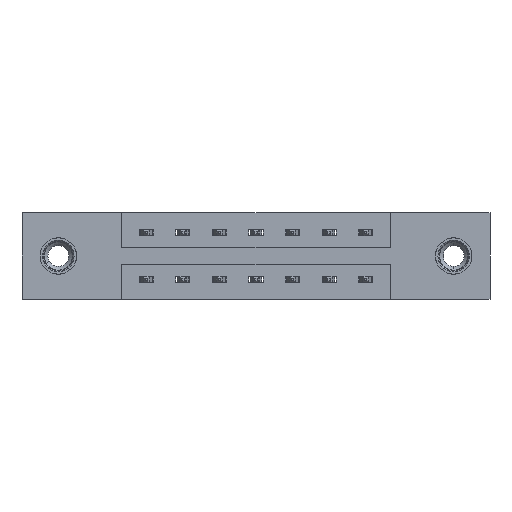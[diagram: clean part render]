
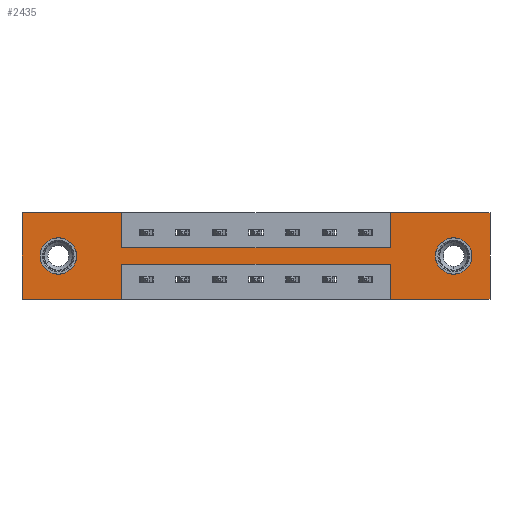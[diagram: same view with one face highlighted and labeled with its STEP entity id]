
A CAD part, front view. The second image highlights one B-rep face of the part: STEP entity #2435.
In plain terms, the highlighted planar face has unit normal (0, -1, 0).
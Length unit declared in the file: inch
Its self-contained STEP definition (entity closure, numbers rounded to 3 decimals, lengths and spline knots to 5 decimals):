
#103 = PLANE ( 'NONE',  #8969 ) ;
#234 = DIRECTION ( 'NONE',  ( 0., 0., 1. ) ) ;
#353 = DIRECTION ( 'NONE',  ( -1., 0., 0. ) ) ;
#356 = CIRCLE ( 'NONE', #10719, 0.078 ) ;
#375 = EDGE_CURVE ( 'NONE', #5994, #7460, #5939, .T. ) ;
#381 = CARTESIAN_POINT ( 'NONE',  ( 0.425, 0., -0.22 ) ) ;
#411 = CARTESIAN_POINT ( 'NONE',  ( 1.843, 0., -0.185 ) ) ;
#418 = EDGE_CURVE ( 'NONE', #3262, #6279, #932, .T. ) ;
#466 = LINE ( 'NONE', #6577, #4883 ) ;
#505 = EDGE_CURVE ( 'NONE', #6763, #5525, #2140, .T. ) ;
#507 = DIRECTION ( 'NONE',  ( 0., -1., 0. ) ) ;
#521 = CARTESIAN_POINT ( 'NONE',  ( 0., 0., -0.37 ) ) ;
#534 = EDGE_CURVE ( 'NONE', #8706, #6865, #11055, .T. ) ;
#595 = AXIS2_PLACEMENT_3D ( 'NONE', #2732, #8881, #3634 ) ;
#843 = EDGE_CURVE ( 'NONE', #5814, #2511, #7992, .T. ) ;
#901 = DIRECTION ( 'NONE',  ( -1., 0., 0. ) ) ;
#932 = LINE ( 'NONE', #4922, #3001 ) ;
#967 = DIRECTION ( 'NONE',  ( 0., 0., -1. ) ) ;
#1188 = VECTOR ( 'NONE', #1465, 39.37008 ) ;
#1202 = CARTESIAN_POINT ( 'NONE',  ( 0.425, 0., -0.15 ) ) ;
#1412 = LINE ( 'NONE', #10168, #8451 ) ;
#1465 = DIRECTION ( 'NONE',  ( -1., 0., 0. ) ) ;
#1551 = CARTESIAN_POINT ( 'NONE',  ( 0., 0., -0.37 ) ) ;
#1708 = ORIENTED_EDGE ( 'NONE', *, *, #534, .F. ) ;
#2140 = CIRCLE ( 'NONE', #7482, 0.078 ) ;
#2142 = CARTESIAN_POINT ( 'NONE',  ( 0., 0., 0. ) ) ;
#2435 = ADVANCED_FACE ( 'NONE', ( #4099, #6209, #8510 ), #103, .T. ) ;
#2511 = VERTEX_POINT ( 'NONE', #2798 ) ;
#2574 = CARTESIAN_POINT ( 'NONE',  ( 1.573, 0., -0.37 ) ) ;
#2670 = LINE ( 'NONE', #7163, #5349 ) ;
#2690 = CARTESIAN_POINT ( 'NONE',  ( 0.155, 0., -0.107 ) ) ;
#2714 = DIRECTION ( 'NONE',  ( 1., 0., 0. ) ) ;
#2716 = EDGE_LOOP ( 'NONE', ( #4762, #5065, #7401, #9607, #5332, #8219, #10369, #10618, #1708, #4637, #6989, #7256 ) ) ;
#2732 = CARTESIAN_POINT ( 'NONE',  ( 0.155, 0., -0.185 ) ) ;
#2735 = VERTEX_POINT ( 'NONE', #2142 ) ;
#2763 = CARTESIAN_POINT ( 'NONE',  ( 0.155, 0., -0.185 ) ) ;
#2777 = DIRECTION ( 'NONE',  ( 0., 0., -1. ) ) ;
#2798 = CARTESIAN_POINT ( 'NONE',  ( 0., 0., -0.37 ) ) ;
#2953 = VERTEX_POINT ( 'NONE', #2690 ) ;
#3001 = VECTOR ( 'NONE', #5689, 39.37008 ) ;
#3045 = VECTOR ( 'NONE', #234, 39.37008 ) ;
#3068 = VERTEX_POINT ( 'NONE', #2574 ) ;
#3210 = CARTESIAN_POINT ( 'NONE',  ( 1.573, 0., -0.15 ) ) ;
#3262 = VERTEX_POINT ( 'NONE', #8260 ) ;
#3384 = DIRECTION ( 'NONE',  ( 0., 0., -1. ) ) ;
#3387 = EDGE_CURVE ( 'NONE', #2735, #8706, #2670, .T. ) ;
#3389 = DIRECTION ( 'NONE',  ( 0., 0., -1. ) ) ;
#3492 = CARTESIAN_POINT ( 'NONE',  ( 0., 0., 0. ) ) ;
#3539 = EDGE_CURVE ( 'NONE', #6865, #8685, #6042, .T. ) ;
#3597 = CIRCLE ( 'NONE', #10507, 0.078 ) ;
#3634 = DIRECTION ( 'NONE',  ( 0., 0., 1. ) ) ;
#3670 = DIRECTION ( 'NONE',  ( 0., 0., 1. ) ) ;
#3967 = EDGE_CURVE ( 'NONE', #7460, #5814, #10506, .T. ) ;
#4099 = FACE_BOUND ( 'NONE', #5236, .T. ) ;
#4181 = CARTESIAN_POINT ( 'NONE',  ( 1.843, 0., -0.185 ) ) ;
#4633 = LINE ( 'NONE', #7412, #11146 ) ;
#4637 = ORIENTED_EDGE ( 'NONE', *, *, #3387, .F. ) ;
#4762 = ORIENTED_EDGE ( 'NONE', *, *, #3967, .F. ) ;
#4883 = VECTOR ( 'NONE', #10585, 39.37008 ) ;
#4922 = CARTESIAN_POINT ( 'NONE',  ( 1.998, 0., 0. ) ) ;
#5016 = CARTESIAN_POINT ( 'NONE',  ( 0.425, 0., -0.15 ) ) ;
#5065 = ORIENTED_EDGE ( 'NONE', *, *, #375, .F. ) ;
#5093 = DIRECTION ( 'NONE',  ( 0., 0., -1. ) ) ;
#5137 = VERTEX_POINT ( 'NONE', #10341 ) ;
#5236 = EDGE_LOOP ( 'NONE', ( #10238, #8347 ) ) ;
#5293 = DIRECTION ( 'NONE',  ( 1., 0., 0. ) ) ;
#5332 = ORIENTED_EDGE ( 'NONE', *, *, #418, .F. ) ;
#5349 = VECTOR ( 'NONE', #2714, 39.37008 ) ;
#5423 = LINE ( 'NONE', #7278, #3045 ) ;
#5525 = VERTEX_POINT ( 'NONE', #6685 ) ;
#5689 = DIRECTION ( 'NONE',  ( 0., 0., -1. ) ) ;
#5747 = EDGE_CURVE ( 'NONE', #2511, #2735, #466, .T. ) ;
#5814 = VERTEX_POINT ( 'NONE', #8512 ) ;
#5864 = EDGE_CURVE ( 'NONE', #3068, #5994, #1412, .T. ) ;
#5939 = LINE ( 'NONE', #381, #10160 ) ;
#5994 = VERTEX_POINT ( 'NONE', #10668 ) ;
#6042 = LINE ( 'NONE', #1202, #10256 ) ;
#6209 = FACE_BOUND ( 'NONE', #8548, .T. ) ;
#6279 = VERTEX_POINT ( 'NONE', #7762 ) ;
#6298 = ORIENTED_EDGE ( 'NONE', *, *, #9656, .T. ) ;
#6348 = VECTOR ( 'NONE', #3389, 39.37008 ) ;
#6543 = CIRCLE ( 'NONE', #595, 0.078 ) ;
#6549 = EDGE_CURVE ( 'NONE', #7294, #2953, #3597, .T. ) ;
#6577 = CARTESIAN_POINT ( 'NONE',  ( 0., 0., 0. ) ) ;
#6606 = EDGE_CURVE ( 'NONE', #8685, #5137, #5423, .T. ) ;
#6631 = CARTESIAN_POINT ( 'NONE',  ( 0.425, 0., -0.22 ) ) ;
#6685 = CARTESIAN_POINT ( 'NONE',  ( 1.843, 0., -0.107 ) ) ;
#6763 = VERTEX_POINT ( 'NONE', #9163 ) ;
#6865 = VERTEX_POINT ( 'NONE', #5016 ) ;
#6989 = ORIENTED_EDGE ( 'NONE', *, *, #5747, .F. ) ;
#7091 = VECTOR ( 'NONE', #5293, 39.37008 ) ;
#7163 = CARTESIAN_POINT ( 'NONE',  ( 0., 0., 0. ) ) ;
#7256 = ORIENTED_EDGE ( 'NONE', *, *, #843, .F. ) ;
#7278 = CARTESIAN_POINT ( 'NONE',  ( 1.573, 0., 0. ) ) ;
#7294 = VERTEX_POINT ( 'NONE', #7301 ) ;
#7301 = CARTESIAN_POINT ( 'NONE',  ( 0.155, 0., -0.263 ) ) ;
#7401 = ORIENTED_EDGE ( 'NONE', *, *, #5864, .F. ) ;
#7412 = CARTESIAN_POINT ( 'NONE',  ( 0., 0., -0.37 ) ) ;
#7416 = DIRECTION ( 'NONE',  ( 0., 1., 0. ) ) ;
#7460 = VERTEX_POINT ( 'NONE', #6631 ) ;
#7482 = AXIS2_PLACEMENT_3D ( 'NONE', #411, #7416, #3384 ) ;
#7762 = CARTESIAN_POINT ( 'NONE',  ( 1.998, 0., -0.37 ) ) ;
#7925 = DIRECTION ( 'NONE',  ( 1., 0., 0. ) ) ;
#7992 = LINE ( 'NONE', #1551, #1188 ) ;
#8062 = CARTESIAN_POINT ( 'NONE',  ( 0.425, 0., -0.37 ) ) ;
#8219 = ORIENTED_EDGE ( 'NONE', *, *, #9571, .F. ) ;
#8260 = CARTESIAN_POINT ( 'NONE',  ( 1.998, 0., 0. ) ) ;
#8347 = ORIENTED_EDGE ( 'NONE', *, *, #505, .T. ) ;
#8451 = VECTOR ( 'NONE', #11130, 39.37008 ) ;
#8493 = CARTESIAN_POINT ( 'NONE',  ( 0.425, 0., 0. ) ) ;
#8510 = FACE_OUTER_BOUND ( 'NONE', #2716, .T. ) ;
#8512 = CARTESIAN_POINT ( 'NONE',  ( 0.425, 0., -0.37 ) ) ;
#8542 = EDGE_CURVE ( 'NONE', #6279, #3068, #4633, .T. ) ;
#8548 = EDGE_LOOP ( 'NONE', ( #6298, #10744 ) ) ;
#8685 = VERTEX_POINT ( 'NONE', #3210 ) ;
#8706 = VERTEX_POINT ( 'NONE', #8493 ) ;
#8735 = EDGE_CURVE ( 'NONE', #5525, #6763, #356, .T. ) ;
#8881 = DIRECTION ( 'NONE',  ( 0., 1., 0. ) ) ;
#8901 = DIRECTION ( 'NONE',  ( 0., 1., 0. ) ) ;
#8969 = AXIS2_PLACEMENT_3D ( 'NONE', #521, #507, #2777 ) ;
#9163 = CARTESIAN_POINT ( 'NONE',  ( 1.843, 0., -0.263 ) ) ;
#9332 = LINE ( 'NONE', #3492, #7091 ) ;
#9571 = EDGE_CURVE ( 'NONE', #5137, #3262, #9332, .T. ) ;
#9607 = ORIENTED_EDGE ( 'NONE', *, *, #8542, .F. ) ;
#9656 = EDGE_CURVE ( 'NONE', #2953, #7294, #6543, .T. ) ;
#10160 = VECTOR ( 'NONE', #901, 39.37008 ) ;
#10168 = CARTESIAN_POINT ( 'NONE',  ( 1.573, 0., -0.37 ) ) ;
#10182 = DIRECTION ( 'NONE',  ( 0., 1., 0. ) ) ;
#10238 = ORIENTED_EDGE ( 'NONE', *, *, #8735, .T. ) ;
#10246 = VECTOR ( 'NONE', #967, 39.37008 ) ;
#10256 = VECTOR ( 'NONE', #7925, 39.37008 ) ;
#10341 = CARTESIAN_POINT ( 'NONE',  ( 1.573, 0., 0. ) ) ;
#10369 = ORIENTED_EDGE ( 'NONE', *, *, #6606, .F. ) ;
#10506 = LINE ( 'NONE', #8062, #10246 ) ;
#10507 = AXIS2_PLACEMENT_3D ( 'NONE', #2763, #8901, #3670 ) ;
#10585 = DIRECTION ( 'NONE',  ( 0., 0., 1. ) ) ;
#10618 = ORIENTED_EDGE ( 'NONE', *, *, #3539, .F. ) ;
#10668 = CARTESIAN_POINT ( 'NONE',  ( 1.573, 0., -0.22 ) ) ;
#10719 = AXIS2_PLACEMENT_3D ( 'NONE', #4181, #10182, #5093 ) ;
#10744 = ORIENTED_EDGE ( 'NONE', *, *, #6549, .T. ) ;
#11045 = CARTESIAN_POINT ( 'NONE',  ( 0.425, 0., 0. ) ) ;
#11055 = LINE ( 'NONE', #11045, #6348 ) ;
#11130 = DIRECTION ( 'NONE',  ( 0., 0., 1. ) ) ;
#11146 = VECTOR ( 'NONE', #353, 39.37008 ) ;
